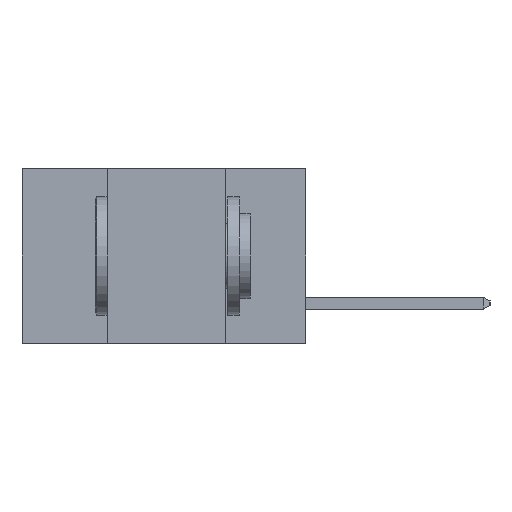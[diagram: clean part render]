
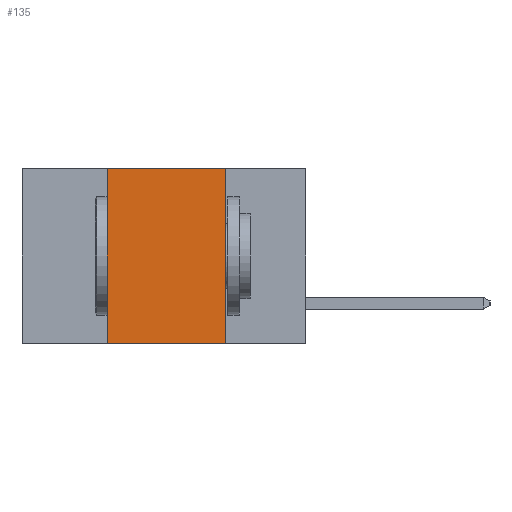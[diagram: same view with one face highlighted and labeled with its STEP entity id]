
A CAD part, left-side view. The second image highlights one B-rep face of the part: STEP entity #135.
In plain terms, the highlighted planar face has unit normal (-1, 0, 0).
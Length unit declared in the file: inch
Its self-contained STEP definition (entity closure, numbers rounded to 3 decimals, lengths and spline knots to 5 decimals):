
#135 = ADVANCED_FACE ( 'NONE', ( #6016 ), #5349, .F. ) ;
#142 = LINE ( 'NONE', #5847, #2086 ) ;
#667 = DIRECTION ( 'NONE',  ( 1., 0., 0. ) ) ;
#690 = CARTESIAN_POINT ( 'NONE',  ( 0., 0.6, 0. ) ) ;
#867 = LINE ( 'NONE', #2191, #8706 ) ;
#1187 = EDGE_CURVE ( 'NONE', #9581, #1359, #9220, .T. ) ;
#1359 = VERTEX_POINT ( 'NONE', #9914 ) ;
#1479 = DIRECTION ( 'NONE',  ( 0., 0., -1. ) ) ;
#1484 = DIRECTION ( 'NONE',  ( 0., 0., 1. ) ) ;
#2086 = VECTOR ( 'NONE', #5941, 39.37008 ) ;
#2165 = ORIENTED_EDGE ( 'NONE', *, *, #4485, .F. ) ;
#2191 = CARTESIAN_POINT ( 'NONE',  ( 0., 0.42, -0.37 ) ) ;
#2332 = CARTESIAN_POINT ( 'NONE',  ( 0., 0.17, -0.37 ) ) ;
#2404 = LINE ( 'NONE', #2332, #2642 ) ;
#2642 = VECTOR ( 'NONE', #3131, 39.37008 ) ;
#3131 = DIRECTION ( 'NONE',  ( 0., 0., -1. ) ) ;
#3174 = DIRECTION ( 'NONE',  ( 0., -1., 0. ) ) ;
#3187 = CARTESIAN_POINT ( 'NONE',  ( 0., 0.42, 0. ) ) ;
#3443 = EDGE_LOOP ( 'NONE', ( #9282, #7530, #2165, #5981 ) ) ;
#4485 = EDGE_CURVE ( 'NONE', #7115, #9581, #867, .T. ) ;
#5031 = CARTESIAN_POINT ( 'NONE',  ( 0., 0.17, -0.37 ) ) ;
#5240 = VECTOR ( 'NONE', #3174, 39.37008 ) ;
#5349 = PLANE ( 'NONE',  #6092 ) ;
#5730 = EDGE_CURVE ( 'NONE', #7115, #9170, #142, .T. ) ;
#5847 = CARTESIAN_POINT ( 'NONE',  ( 0., 0.6, -0.37 ) ) ;
#5941 = DIRECTION ( 'NONE',  ( 0., -1., 0. ) ) ;
#5981 = ORIENTED_EDGE ( 'NONE', *, *, #5730, .T. ) ;
#6016 = FACE_OUTER_BOUND ( 'NONE', #3443, .T. ) ;
#6092 = AXIS2_PLACEMENT_3D ( 'NONE', #6229, #667, #1479 ) ;
#6229 = CARTESIAN_POINT ( 'NONE',  ( 0., 0.6, 0. ) ) ;
#7092 = EDGE_CURVE ( 'NONE', #1359, #9170, #2404, .T. ) ;
#7115 = VERTEX_POINT ( 'NONE', #7902 ) ;
#7530 = ORIENTED_EDGE ( 'NONE', *, *, #1187, .F. ) ;
#7902 = CARTESIAN_POINT ( 'NONE',  ( 0., 0.42, -0.37 ) ) ;
#8706 = VECTOR ( 'NONE', #1484, 39.37008 ) ;
#9170 = VERTEX_POINT ( 'NONE', #5031 ) ;
#9220 = LINE ( 'NONE', #690, #5240 ) ;
#9282 = ORIENTED_EDGE ( 'NONE', *, *, #7092, .F. ) ;
#9581 = VERTEX_POINT ( 'NONE', #3187 ) ;
#9914 = CARTESIAN_POINT ( 'NONE',  ( 0., 0.17, 0. ) ) ;
